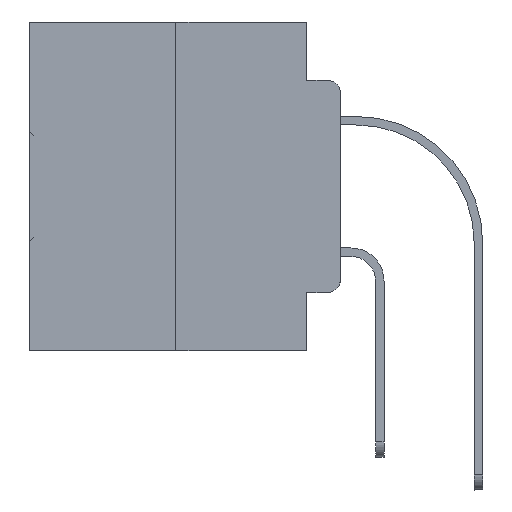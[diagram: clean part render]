
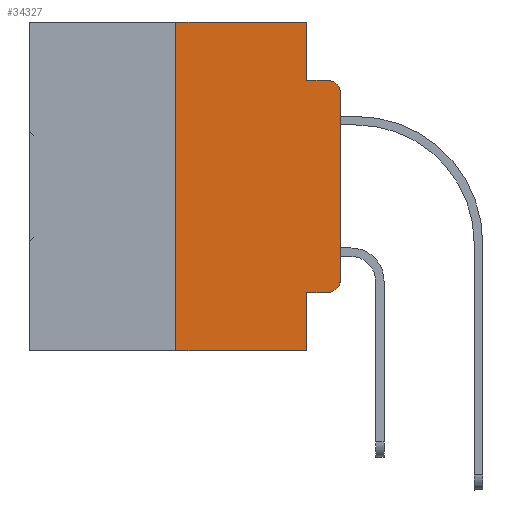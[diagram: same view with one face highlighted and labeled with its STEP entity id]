
A CAD part, left-side view. The second image highlights one B-rep face of the part: STEP entity #34327.
In plain terms, the highlighted planar face has unit normal (-1, 0, 0).
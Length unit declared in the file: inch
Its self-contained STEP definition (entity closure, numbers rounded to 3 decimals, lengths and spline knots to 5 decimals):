
#332 = AXIS2_PLACEMENT_3D ( 'NONE', #29687, #30212, #27404 ) ;
#527 = DIRECTION ( 'NONE',  ( 0., -1., 0. ) ) ;
#2362 = VERTEX_POINT ( 'NONE', #6818 ) ;
#2614 = CARTESIAN_POINT ( 'NONE',  ( 0., 0.25, 0. ) ) ;
#3559 = ORIENTED_EDGE ( 'NONE', *, *, #12226, .F. ) ;
#4002 = LINE ( 'NONE', #17660, #20059 ) ;
#4923 = AXIS2_PLACEMENT_3D ( 'NONE', #20088, #19231, #27179 ) ;
#5328 = LINE ( 'NONE', #16508, #29703 ) ;
#5842 = EDGE_CURVE ( 'NONE', #29936, #17442, #16271, .T. ) ;
#6053 = CARTESIAN_POINT ( 'NONE',  ( 0., 0.473, 0. ) ) ;
#6202 = CARTESIAN_POINT ( 'NONE',  ( 0., 0.02, -0.3915 ) ) ;
#6579 = CARTESIAN_POINT ( 'NONE',  ( 0., 0.051, -0.4115 ) ) ;
#6818 = CARTESIAN_POINT ( 'NONE',  ( 0., 0.051, 0. ) ) ;
#6883 = VERTEX_POINT ( 'NONE', #22391 ) ;
#7262 = VERTEX_POINT ( 'NONE', #26415 ) ;
#7347 = VECTOR ( 'NONE', #527, 39.37008 ) ;
#8725 = ORIENTED_EDGE ( 'NONE', *, *, #16467, .T. ) ;
#9990 = DIRECTION ( 'NONE',  ( 0., -1., 0. ) ) ;
#10007 = CARTESIAN_POINT ( 'NONE',  ( 0., 0.02, -0.0885 ) ) ;
#10199 = DIRECTION ( 'NONE',  ( 0., 0., 1. ) ) ;
#10807 = EDGE_LOOP ( 'NONE', ( #15767, #16241, #18604, #32686, #3559, #25195, #8725, #22884, #15928, #26886 ) ) ;
#11102 = FACE_OUTER_BOUND ( 'NONE', #10807, .T. ) ;
#12226 = EDGE_CURVE ( 'NONE', #17442, #2362, #33125, .T. ) ;
#12581 = VERTEX_POINT ( 'NONE', #13513 ) ;
#12991 = LINE ( 'NONE', #26603, #27326 ) ;
#13105 = VERTEX_POINT ( 'NONE', #24796 ) ;
#13513 = CARTESIAN_POINT ( 'NONE',  ( 0., 0.051, -0.4115 ) ) ;
#14392 = DIRECTION ( 'NONE',  ( 0., 0., -1. ) ) ;
#15014 = LINE ( 'NONE', #33891, #28523 ) ;
#15538 = VECTOR ( 'NONE', #9990, 39.37008 ) ;
#15767 = ORIENTED_EDGE ( 'NONE', *, *, #23254, .T. ) ;
#15928 = ORIENTED_EDGE ( 'NONE', *, *, #19630, .T. ) ;
#16241 = ORIENTED_EDGE ( 'NONE', *, *, #32894, .T. ) ;
#16271 = LINE ( 'NONE', #2614, #23958 ) ;
#16462 = CARTESIAN_POINT ( 'NONE',  ( 0., 0., -0.3915 ) ) ;
#16467 = EDGE_CURVE ( 'NONE', #29936, #6883, #28913, .T. ) ;
#16508 = CARTESIAN_POINT ( 'NONE',  ( 0., 0.051, 0. ) ) ;
#17031 = DIRECTION ( 'NONE',  ( -1., 0., 0. ) ) ;
#17442 = VERTEX_POINT ( 'NONE', #21948 ) ;
#17660 = CARTESIAN_POINT ( 'NONE',  ( 0., 0., 0. ) ) ;
#18604 = ORIENTED_EDGE ( 'NONE', *, *, #27248, .F. ) ;
#18846 = VERTEX_POINT ( 'NONE', #16462 ) ;
#19231 = DIRECTION ( 'NONE',  ( 1., 0., 0. ) ) ;
#19630 = EDGE_CURVE ( 'NONE', #12581, #13105, #27832, .T. ) ;
#19706 = DIRECTION ( 'NONE',  ( 0., -1., 0. ) ) ;
#20059 = VECTOR ( 'NONE', #10199, 39.37008 ) ;
#20088 = CARTESIAN_POINT ( 'NONE',  ( 0., 0.473, 0. ) ) ;
#20459 = VECTOR ( 'NONE', #19706, 39.37008 ) ;
#20709 = AXIS2_PLACEMENT_3D ( 'NONE', #6202, #17031, #14392 ) ;
#21010 = DIRECTION ( 'NONE',  ( 0., 0., -1. ) ) ;
#21407 = DIRECTION ( 'NONE',  ( 0., 0., 1. ) ) ;
#21948 = CARTESIAN_POINT ( 'NONE',  ( 0., 0.25, 0. ) ) ;
#22391 = CARTESIAN_POINT ( 'NONE',  ( 0., 0.051, -0.5 ) ) ;
#22415 = CIRCLE ( 'NONE', #20709, 0.02 ) ;
#22884 = ORIENTED_EDGE ( 'NONE', *, *, #30664, .F. ) ;
#23254 = EDGE_CURVE ( 'NONE', #18846, #29229, #4002, .T. ) ;
#23273 = EDGE_CURVE ( 'NONE', #2362, #7262, #15014, .T. ) ;
#23441 = CARTESIAN_POINT ( 'NONE',  ( 0., 0.473, -0.5 ) ) ;
#23958 = VECTOR ( 'NONE', #21407, 39.37008 ) ;
#24796 = CARTESIAN_POINT ( 'NONE',  ( 0., 0.02, -0.4115 ) ) ;
#25195 = ORIENTED_EDGE ( 'NONE', *, *, #5842, .F. ) ;
#26415 = CARTESIAN_POINT ( 'NONE',  ( 0., 0.051, -0.0885 ) ) ;
#26603 = CARTESIAN_POINT ( 'NONE',  ( 0., 0.051, -0.0885 ) ) ;
#26886 = ORIENTED_EDGE ( 'NONE', *, *, #30867, .T. ) ;
#27179 = DIRECTION ( 'NONE',  ( 0., 0., -1. ) ) ;
#27248 = EDGE_CURVE ( 'NONE', #7262, #28409, #12991, .T. ) ;
#27302 = DIRECTION ( 'NONE',  ( 0., 0., -1. ) ) ;
#27326 = VECTOR ( 'NONE', #34741, 39.37008 ) ;
#27404 = DIRECTION ( 'NONE',  ( 0., 0., -1. ) ) ;
#27832 = LINE ( 'NONE', #6579, #20459 ) ;
#28369 = PLANE ( 'NONE',  #4923 ) ;
#28409 = VERTEX_POINT ( 'NONE', #10007 ) ;
#28523 = VECTOR ( 'NONE', #21010, 39.37008 ) ;
#28913 = LINE ( 'NONE', #23441, #15538 ) ;
#29229 = VERTEX_POINT ( 'NONE', #29386 ) ;
#29386 = CARTESIAN_POINT ( 'NONE',  ( 0., 0., -0.1085 ) ) ;
#29687 = CARTESIAN_POINT ( 'NONE',  ( 0., 0.02, -0.1085 ) ) ;
#29703 = VECTOR ( 'NONE', #27302, 39.37008 ) ;
#29936 = VERTEX_POINT ( 'NONE', #32870 ) ;
#30212 = DIRECTION ( 'NONE',  ( -1., 0., 0. ) ) ;
#30664 = EDGE_CURVE ( 'NONE', #12581, #6883, #5328, .T. ) ;
#30867 = EDGE_CURVE ( 'NONE', #13105, #18846, #22415, .T. ) ;
#32686 = ORIENTED_EDGE ( 'NONE', *, *, #23273, .F. ) ;
#32870 = CARTESIAN_POINT ( 'NONE',  ( 0., 0.25, -0.5 ) ) ;
#32894 = EDGE_CURVE ( 'NONE', #29229, #28409, #33133, .T. ) ;
#33125 = LINE ( 'NONE', #6053, #7347 ) ;
#33133 = CIRCLE ( 'NONE', #332, 0.02 ) ;
#33891 = CARTESIAN_POINT ( 'NONE',  ( 0., 0.051, 0. ) ) ;
#34327 = ADVANCED_FACE ( 'NONE', ( #11102 ), #28369, .F. ) ;
#34741 = DIRECTION ( 'NONE',  ( 0., -1., 0. ) ) ;
